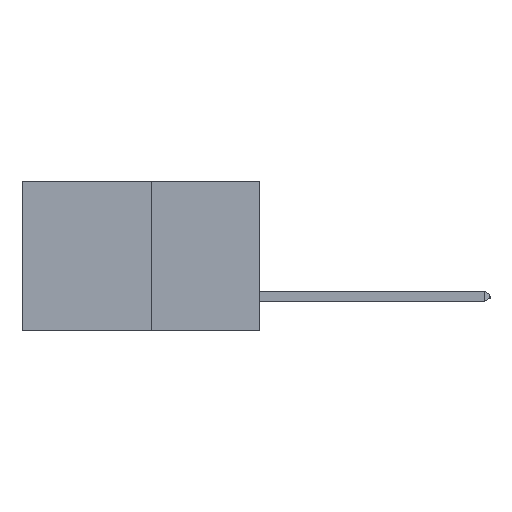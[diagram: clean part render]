
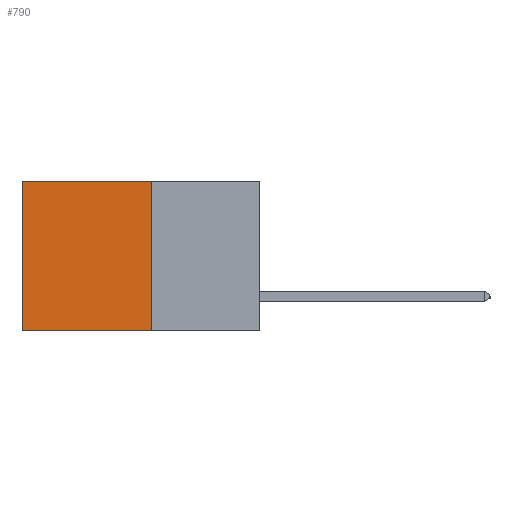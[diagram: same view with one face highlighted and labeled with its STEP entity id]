
A CAD part, left-side view. The second image highlights one B-rep face of the part: STEP entity #790.
In plain terms, the highlighted planar face has unit normal (-1, 0, 0).
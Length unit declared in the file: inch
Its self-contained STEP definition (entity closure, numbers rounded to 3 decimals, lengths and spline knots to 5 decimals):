
#301 = ORIENTED_EDGE ( 'NONE', *, *, #4757, .F. ) ;
#357 = CARTESIAN_POINT ( 'NONE',  ( 0.277, 0.27, -0.37 ) ) ;
#660 = LINE ( 'NONE', #8263, #10922 ) ;
#790 = ADVANCED_FACE ( 'NONE', ( #6083 ), #3403, .F. ) ;
#1412 = CARTESIAN_POINT ( 'NONE',  ( 0.277, 0.59, 0. ) ) ;
#1738 = LINE ( 'NONE', #7184, #4080 ) ;
#1780 = EDGE_CURVE ( 'NONE', #4604, #3021, #12768, .T. ) ;
#2355 = DIRECTION ( 'NONE',  ( 0., 0., -1. ) ) ;
#3021 = VERTEX_POINT ( 'NONE', #4029 ) ;
#3098 = DIRECTION ( 'NONE',  ( 1., 0., 0. ) ) ;
#3138 = DIRECTION ( 'NONE',  ( 0., 0., -1. ) ) ;
#3145 = CARTESIAN_POINT ( 'NONE',  ( 0.277, 0.27, 0. ) ) ;
#3403 = PLANE ( 'NONE',  #9696 ) ;
#3767 = EDGE_LOOP ( 'NONE', ( #9670, #4852, #301, #5553 ) ) ;
#3884 = EDGE_CURVE ( 'NONE', #8166, #4604, #4722, .T. ) ;
#4029 = CARTESIAN_POINT ( 'NONE',  ( 0.277, 0.59, -0.37 ) ) ;
#4080 = VECTOR ( 'NONE', #3138, 39.37008 ) ;
#4265 = CARTESIAN_POINT ( 'NONE',  ( 0.277, 0.59, -0.37 ) ) ;
#4295 = DIRECTION ( 'NONE',  ( 0., 1., 0. ) ) ;
#4604 = VERTEX_POINT ( 'NONE', #1412 ) ;
#4667 = CARTESIAN_POINT ( 'NONE',  ( 0.277, 0.27, -0.37 ) ) ;
#4722 = LINE ( 'NONE', #10481, #11361 ) ;
#4757 = EDGE_CURVE ( 'NONE', #8166, #5135, #1738, .T. ) ;
#4852 = ORIENTED_EDGE ( 'NONE', *, *, #11553, .F. ) ;
#5135 = VERTEX_POINT ( 'NONE', #4667 ) ;
#5553 = ORIENTED_EDGE ( 'NONE', *, *, #3884, .T. ) ;
#6083 = FACE_OUTER_BOUND ( 'NONE', #3767, .T. ) ;
#7184 = CARTESIAN_POINT ( 'NONE',  ( 0.277, 0.27, -0.37 ) ) ;
#7344 = VECTOR ( 'NONE', #11838, 39.37008 ) ;
#8005 = DIRECTION ( 'NONE',  ( 0., 1., 0. ) ) ;
#8166 = VERTEX_POINT ( 'NONE', #3145 ) ;
#8263 = CARTESIAN_POINT ( 'NONE',  ( 0.277, 0.27, -0.37 ) ) ;
#9670 = ORIENTED_EDGE ( 'NONE', *, *, #1780, .T. ) ;
#9696 = AXIS2_PLACEMENT_3D ( 'NONE', #357, #3098, #2355 ) ;
#10481 = CARTESIAN_POINT ( 'NONE',  ( 0.277, 0.27, 0. ) ) ;
#10922 = VECTOR ( 'NONE', #4295, 39.37008 ) ;
#11361 = VECTOR ( 'NONE', #8005, 39.37008 ) ;
#11553 = EDGE_CURVE ( 'NONE', #5135, #3021, #660, .T. ) ;
#11838 = DIRECTION ( 'NONE',  ( 0., 0., -1. ) ) ;
#12768 = LINE ( 'NONE', #4265, #7344 ) ;
